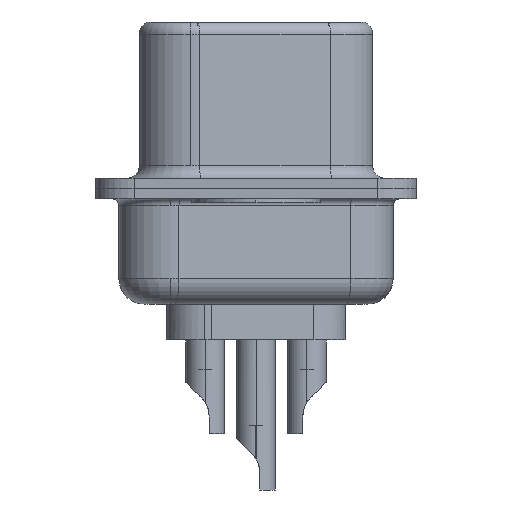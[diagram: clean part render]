
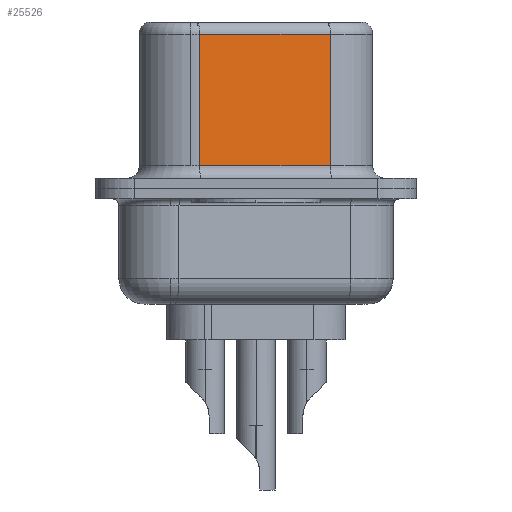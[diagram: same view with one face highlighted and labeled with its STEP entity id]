
A CAD part, left-side view. The second image highlights one B-rep face of the part: STEP entity #25526.
In plain terms, the highlighted planar face has unit normal (-0.985, -0.174, 0).
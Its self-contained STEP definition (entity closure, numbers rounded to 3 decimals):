
#687 = FACE_OUTER_BOUND ( 'NONE', #28790, .T. ) ;
#823 = CARTESIAN_POINT ( 'NONE',  ( 4.58, -2.897, 0.9 ) ) ;
#1920 = DIRECTION ( 'NONE',  ( 0.174, -0.985, 0. ) ) ;
#1928 = DIRECTION ( 'NONE',  ( 0.985, 0.174, 0. ) ) ;
#3470 = LINE ( 'NONE', #22547, #21739 ) ;
#3591 = CARTESIAN_POINT ( 'NONE',  ( 4.58, -2.897, 6.02 ) ) ;
#4782 = VERTEX_POINT ( 'NONE', #823 ) ;
#5396 = ORIENTED_EDGE ( 'NONE', *, *, #10039, .T. ) ;
#8841 = VERTEX_POINT ( 'NONE', #3591 ) ;
#10039 = EDGE_CURVE ( 'NONE', #8841, #14613, #13504, .T. ) ;
#11516 = CARTESIAN_POINT ( 'NONE',  ( 4.58, -2.897, 0.9 ) ) ;
#12740 = CARTESIAN_POINT ( 'NONE',  ( 3.68, 2.203, 0.9 ) ) ;
#13504 = LINE ( 'NONE', #28217, #19773 ) ;
#14077 = DIRECTION ( 'NONE',  ( -0.174, 0.985, 0. ) ) ;
#14613 = VERTEX_POINT ( 'NONE', #18515 ) ;
#15391 = LINE ( 'NONE', #11516, #27952 ) ;
#15809 = CARTESIAN_POINT ( 'NONE',  ( 3.68, 2.203, 6.52 ) ) ;
#17599 = LINE ( 'NONE', #15809, #23035 ) ;
#18204 = DIRECTION ( 'NONE',  ( 0., 0., -1. ) ) ;
#18515 = CARTESIAN_POINT ( 'NONE',  ( 3.68, 2.203, 6.02 ) ) ;
#18686 = DIRECTION ( 'NONE',  ( -0.174, 0.985, 0. ) ) ;
#18791 = EDGE_CURVE ( 'NONE', #27620, #4782, #15391, .T. ) ;
#19773 = VECTOR ( 'NONE', #14077, 1000. ) ;
#21739 = VECTOR ( 'NONE', #27372, 1000. ) ;
#22331 = ORIENTED_EDGE ( 'NONE', *, *, #23473, .F. ) ;
#22547 = CARTESIAN_POINT ( 'NONE',  ( 4.58, -2.897, 6.52 ) ) ;
#23035 = VECTOR ( 'NONE', #18204, 1000. ) ;
#23473 = EDGE_CURVE ( 'NONE', #8841, #4782, #3470, .T. ) ;
#25526 = ADVANCED_FACE ( 'NONE', ( #687 ), #30441, .F. ) ;
#25539 = AXIS2_PLACEMENT_3D ( 'NONE', #25654, #1928, #18686 ) ;
#25654 = CARTESIAN_POINT ( 'NONE',  ( 4.58, -2.897, 6.52 ) ) ;
#27372 = DIRECTION ( 'NONE',  ( 0., 0., -1. ) ) ;
#27620 = VERTEX_POINT ( 'NONE', #12740 ) ;
#27952 = VECTOR ( 'NONE', #1920, 1000. ) ;
#28217 = CARTESIAN_POINT ( 'NONE',  ( 4.58, -2.897, 6.02 ) ) ;
#28790 = EDGE_LOOP ( 'NONE', ( #22331, #5396, #29832, #30423 ) ) ;
#29741 = EDGE_CURVE ( 'NONE', #14613, #27620, #17599, .T. ) ;
#29832 = ORIENTED_EDGE ( 'NONE', *, *, #29741, .T. ) ;
#30423 = ORIENTED_EDGE ( 'NONE', *, *, #18791, .T. ) ;
#30441 = PLANE ( 'NONE',  #25539 ) ;
